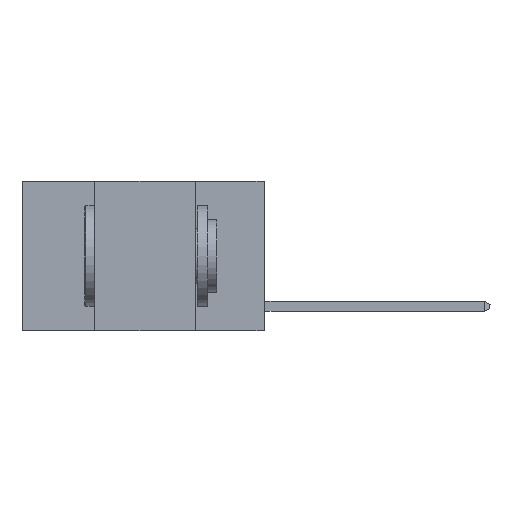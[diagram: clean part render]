
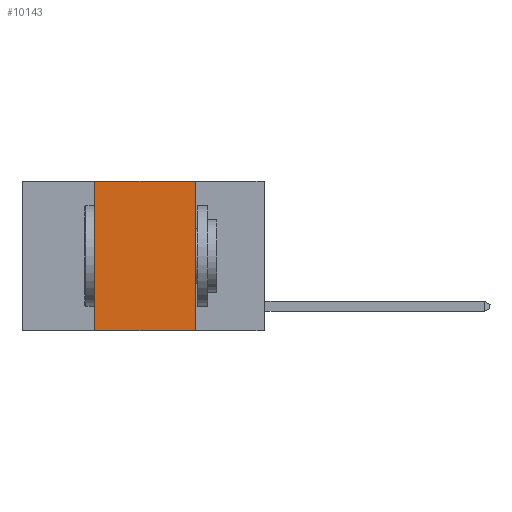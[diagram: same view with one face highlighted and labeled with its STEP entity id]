
A CAD part, left-side view. The second image highlights one B-rep face of the part: STEP entity #10143.
In plain terms, the highlighted planar face has unit normal (-1, 0, 0).
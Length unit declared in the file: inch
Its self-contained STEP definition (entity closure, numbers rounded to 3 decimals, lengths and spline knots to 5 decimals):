
#202 = VECTOR ( 'NONE', #15331, 39.37008 ) ;
#253 = LINE ( 'NONE', #16647, #13488 ) ;
#697 = ORIENTED_EDGE ( 'NONE', *, *, #8123, .F. ) ;
#1037 = DIRECTION ( 'NONE',  ( 0., -1., 0. ) ) ;
#1296 = VERTEX_POINT ( 'NONE', #8275 ) ;
#2775 = CARTESIAN_POINT ( 'NONE',  ( 0., 0.6, 0. ) ) ;
#3500 = DIRECTION ( 'NONE',  ( 0., 0., 1. ) ) ;
#4057 = DIRECTION ( 'NONE',  ( 0., 0., -1. ) ) ;
#4143 = DIRECTION ( 'NONE',  ( 1., 0., 0. ) ) ;
#4793 = ORIENTED_EDGE ( 'NONE', *, *, #17835, .F. ) ;
#5227 = CARTESIAN_POINT ( 'NONE',  ( 0., 0.17, 0. ) ) ;
#6149 = EDGE_LOOP ( 'NONE', ( #697, #4793, #16159, #14321 ) ) ;
#6282 = EDGE_CURVE ( 'NONE', #12037, #15859, #253, .T. ) ;
#6317 = CARTESIAN_POINT ( 'NONE',  ( 0., 0.17, -0.37 ) ) ;
#6600 = VECTOR ( 'NONE', #9591, 39.37008 ) ;
#8123 = EDGE_CURVE ( 'NONE', #1296, #8924, #8414, .T. ) ;
#8275 = CARTESIAN_POINT ( 'NONE',  ( 0., 0.17, 0. ) ) ;
#8295 = LINE ( 'NONE', #15714, #202 ) ;
#8414 = LINE ( 'NONE', #5227, #6600 ) ;
#8571 = CARTESIAN_POINT ( 'NONE',  ( 0., 0.6, 0. ) ) ;
#8814 = AXIS2_PLACEMENT_3D ( 'NONE', #2775, #4143, #4057 ) ;
#8924 = VERTEX_POINT ( 'NONE', #6317 ) ;
#9591 = DIRECTION ( 'NONE',  ( 0., 0., -1. ) ) ;
#10143 = ADVANCED_FACE ( 'NONE', ( #18803 ), #15899, .F. ) ;
#11399 = EDGE_CURVE ( 'NONE', #12037, #8924, #8295, .T. ) ;
#12037 = VERTEX_POINT ( 'NONE', #13555 ) ;
#12119 = CARTESIAN_POINT ( 'NONE',  ( 0., 0.42, 0. ) ) ;
#13488 = VECTOR ( 'NONE', #3500, 39.37008 ) ;
#13555 = CARTESIAN_POINT ( 'NONE',  ( 0., 0.42, -0.37 ) ) ;
#14254 = LINE ( 'NONE', #8571, #16977 ) ;
#14321 = ORIENTED_EDGE ( 'NONE', *, *, #11399, .T. ) ;
#15331 = DIRECTION ( 'NONE',  ( 0., -1., 0. ) ) ;
#15714 = CARTESIAN_POINT ( 'NONE',  ( 0., 0.6, -0.37 ) ) ;
#15859 = VERTEX_POINT ( 'NONE', #12119 ) ;
#15899 = PLANE ( 'NONE',  #8814 ) ;
#16159 = ORIENTED_EDGE ( 'NONE', *, *, #6282, .F. ) ;
#16647 = CARTESIAN_POINT ( 'NONE',  ( 0., 0.42, 0. ) ) ;
#16977 = VECTOR ( 'NONE', #1037, 39.37008 ) ;
#17835 = EDGE_CURVE ( 'NONE', #15859, #1296, #14254, .T. ) ;
#18803 = FACE_OUTER_BOUND ( 'NONE', #6149, .T. ) ;
